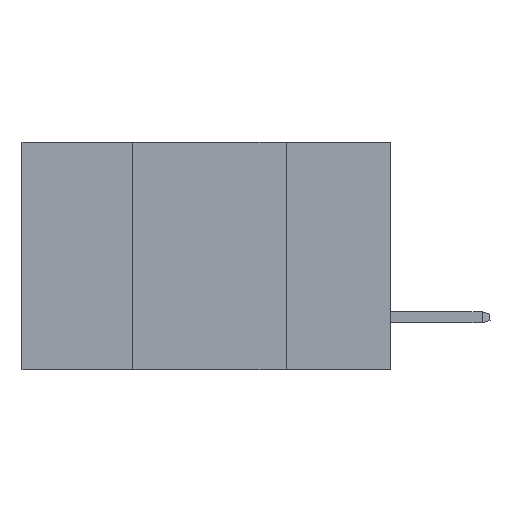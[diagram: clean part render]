
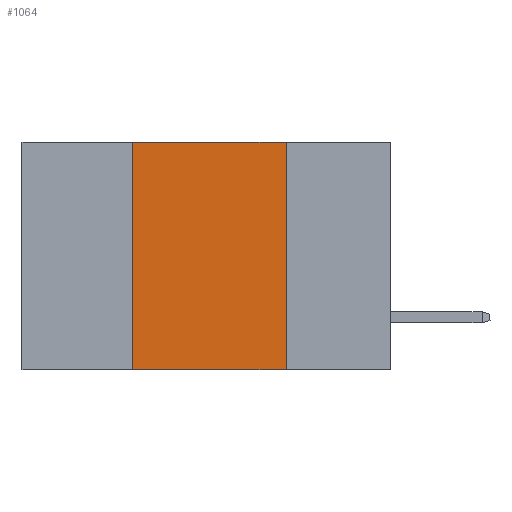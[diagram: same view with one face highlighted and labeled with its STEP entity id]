
A CAD part, left-side view. The second image highlights one B-rep face of the part: STEP entity #1064.
In plain terms, the highlighted planar face has unit normal (-1, 0, 0).
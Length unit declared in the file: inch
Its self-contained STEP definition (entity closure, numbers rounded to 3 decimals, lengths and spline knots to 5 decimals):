
#1064 = ADVANCED_FACE ( 'NONE', ( #4400 ), #2474, .F. ) ;
#1476 = CARTESIAN_POINT ( 'NONE',  ( 0., 0.42, 0. ) ) ;
#1493 = VERTEX_POINT ( 'NONE', #9777 ) ;
#1948 = LINE ( 'NONE', #2195, #7127 ) ;
#2195 = CARTESIAN_POINT ( 'NONE',  ( 0., 0.42, 0. ) ) ;
#2419 = ORIENTED_EDGE ( 'NONE', *, *, #11287, .F. ) ;
#2474 = PLANE ( 'NONE',  #9722 ) ;
#2525 = ORIENTED_EDGE ( 'NONE', *, *, #8846, .F. ) ;
#2899 = DIRECTION ( 'NONE',  ( 1., 0., 0. ) ) ;
#3702 = EDGE_CURVE ( 'NONE', #1493, #8411, #9944, .T. ) ;
#4400 = FACE_OUTER_BOUND ( 'NONE', #5224, .T. ) ;
#5224 = EDGE_LOOP ( 'NONE', ( #5476, #2525, #2419, #10752 ) ) ;
#5476 = ORIENTED_EDGE ( 'NONE', *, *, #3702, .F. ) ;
#6290 = CARTESIAN_POINT ( 'NONE',  ( 0., 0.6, 0. ) ) ;
#6315 = DIRECTION ( 'NONE',  ( 0., 0., 1. ) ) ;
#7127 = VECTOR ( 'NONE', #6315, 39.37008 ) ;
#7189 = CARTESIAN_POINT ( 'NONE',  ( 0., 0.42, -0.37 ) ) ;
#8320 = DIRECTION ( 'NONE',  ( 0., 0., -1. ) ) ;
#8407 = CARTESIAN_POINT ( 'NONE',  ( 0., 0.17, 0. ) ) ;
#8411 = VERTEX_POINT ( 'NONE', #13182 ) ;
#8413 = VECTOR ( 'NONE', #11881, 39.37008 ) ;
#8846 = EDGE_CURVE ( 'NONE', #12993, #1493, #11464, .T. ) ;
#9002 = VECTOR ( 'NONE', #11836, 39.37008 ) ;
#9318 = LINE ( 'NONE', #10825, #9002 ) ;
#9722 = AXIS2_PLACEMENT_3D ( 'NONE', #6290, #2899, #12981 ) ;
#9739 = VERTEX_POINT ( 'NONE', #7189 ) ;
#9777 = CARTESIAN_POINT ( 'NONE',  ( 0., 0.17, 0. ) ) ;
#9861 = CARTESIAN_POINT ( 'NONE',  ( 0., 0.6, 0. ) ) ;
#9944 = LINE ( 'NONE', #8407, #12599 ) ;
#10752 = ORIENTED_EDGE ( 'NONE', *, *, #11528, .T. ) ;
#10825 = CARTESIAN_POINT ( 'NONE',  ( 0., 0.6, -0.37 ) ) ;
#11287 = EDGE_CURVE ( 'NONE', #9739, #12993, #1948, .T. ) ;
#11464 = LINE ( 'NONE', #9861, #8413 ) ;
#11528 = EDGE_CURVE ( 'NONE', #9739, #8411, #9318, .T. ) ;
#11836 = DIRECTION ( 'NONE',  ( 0., -1., 0. ) ) ;
#11881 = DIRECTION ( 'NONE',  ( 0., -1., 0. ) ) ;
#12599 = VECTOR ( 'NONE', #8320, 39.37008 ) ;
#12981 = DIRECTION ( 'NONE',  ( 0., 0., -1. ) ) ;
#12993 = VERTEX_POINT ( 'NONE', #1476 ) ;
#13182 = CARTESIAN_POINT ( 'NONE',  ( 0., 0.17, -0.37 ) ) ;
